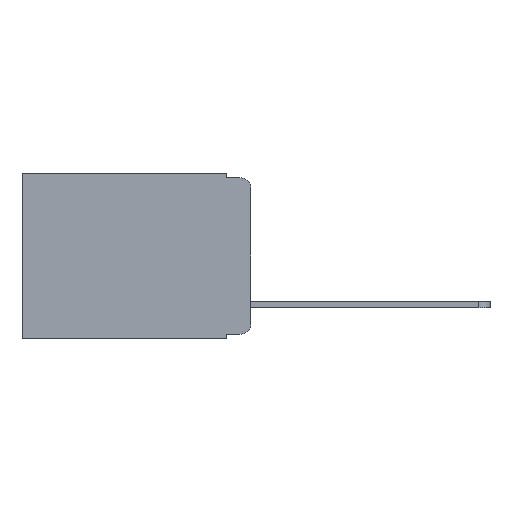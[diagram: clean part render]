
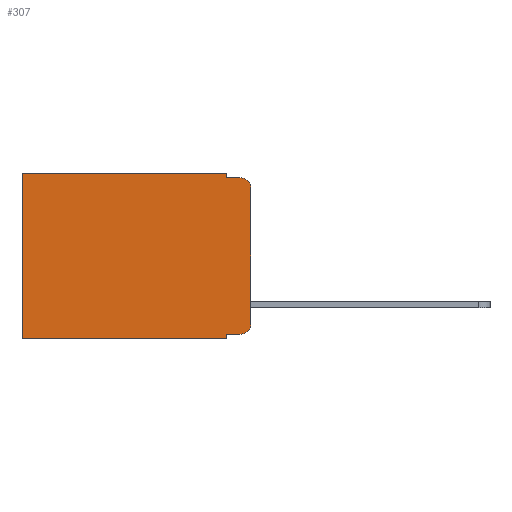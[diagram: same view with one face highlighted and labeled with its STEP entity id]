
A CAD part, left-side view. The second image highlights one B-rep face of the part: STEP entity #307.
In plain terms, the highlighted planar face has unit normal (-1, 0, 0).
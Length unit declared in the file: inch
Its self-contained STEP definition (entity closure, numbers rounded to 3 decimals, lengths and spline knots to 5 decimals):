
#84 = VERTEX_POINT ( 'NONE', #14097 ) ;
#109 = CARTESIAN_POINT ( 'NONE',  ( 0.298, 0.051, -0.01 ) ) ;
#186 = DIRECTION ( 'NONE',  ( 0., 0., -1. ) ) ;
#307 = ADVANCED_FACE ( 'NONE', ( #3112 ), #5571, .F. ) ;
#440 = VERTEX_POINT ( 'NONE', #2678 ) ;
#687 = CARTESIAN_POINT ( 'NONE',  ( 0.298, 0.051, -0.333 ) ) ;
#953 = AXIS2_PLACEMENT_3D ( 'NONE', #9244, #13733, #14903 ) ;
#974 = CARTESIAN_POINT ( 'NONE',  ( 0.298, 0., 0. ) ) ;
#1212 = DIRECTION ( 'NONE',  ( -1., 0., 0. ) ) ;
#1308 = EDGE_CURVE ( 'NONE', #11328, #84, #1599, .T. ) ;
#1599 = LINE ( 'NONE', #687, #10587 ) ;
#1631 = EDGE_CURVE ( 'NONE', #14155, #2158, #12744, .T. ) ;
#1841 = CARTESIAN_POINT ( 'NONE',  ( 0.298, 0.051, 0. ) ) ;
#2158 = VERTEX_POINT ( 'NONE', #7112 ) ;
#2267 = DIRECTION ( 'NONE',  ( 0., 1., 0. ) ) ;
#2623 = EDGE_LOOP ( 'NONE', ( #8849, #6569, #5108, #6076, #7747, #9225, #6138, #6035, #11601, #13265 ) ) ;
#2652 = CARTESIAN_POINT ( 'NONE',  ( 0.298, 0., -0.03 ) ) ;
#2678 = CARTESIAN_POINT ( 'NONE',  ( 0.298, 0.051, -0.01 ) ) ;
#2865 = VECTOR ( 'NONE', #2267, 39.37008 ) ;
#3112 = FACE_OUTER_BOUND ( 'NONE', #2623, .T. ) ;
#3610 = LINE ( 'NONE', #4688, #4541 ) ;
#3996 = EDGE_CURVE ( 'NONE', #10673, #12956, #5296, .T. ) ;
#4031 = VECTOR ( 'NONE', #14235, 39.37008 ) ;
#4123 = CARTESIAN_POINT ( 'NONE',  ( 0.298, 0., -0.313 ) ) ;
#4240 = VERTEX_POINT ( 'NONE', #4123 ) ;
#4541 = VECTOR ( 'NONE', #186, 39.37008 ) ;
#4688 = CARTESIAN_POINT ( 'NONE',  ( 0.298, 0.051, 0. ) ) ;
#4751 = EDGE_CURVE ( 'NONE', #11328, #10673, #3610, .T. ) ;
#4958 = EDGE_CURVE ( 'NONE', #12602, #440, #14024, .T. ) ;
#5108 = ORIENTED_EDGE ( 'NONE', *, *, #14728, .F. ) ;
#5249 = LINE ( 'NONE', #109, #7482 ) ;
#5296 = LINE ( 'NONE', #10644, #13701 ) ;
#5571 = PLANE ( 'NONE',  #953 ) ;
#5647 = CARTESIAN_POINT ( 'NONE',  ( 0.298, 0.051, 0. ) ) ;
#5767 = VECTOR ( 'NONE', #6922, 39.37008 ) ;
#5869 = CARTESIAN_POINT ( 'NONE',  ( 0.298, 0.02, -0.03 ) ) ;
#5973 = EDGE_CURVE ( 'NONE', #5981, #12956, #7658, .T. ) ;
#5981 = VERTEX_POINT ( 'NONE', #11500 ) ;
#6035 = ORIENTED_EDGE ( 'NONE', *, *, #4751, .F. ) ;
#6076 = ORIENTED_EDGE ( 'NONE', *, *, #4958, .F. ) ;
#6138 = ORIENTED_EDGE ( 'NONE', *, *, #3996, .F. ) ;
#6381 = EDGE_CURVE ( 'NONE', #12602, #5981, #12183, .T. ) ;
#6569 = ORIENTED_EDGE ( 'NONE', *, *, #1631, .T. ) ;
#6681 = AXIS2_PLACEMENT_3D ( 'NONE', #5869, #1212, #10533 ) ;
#6922 = DIRECTION ( 'NONE',  ( 0., 0., -1. ) ) ;
#6939 = CARTESIAN_POINT ( 'NONE',  ( 0.298, 0.473, -0.343 ) ) ;
#6941 = DIRECTION ( 'NONE',  ( 0., 0., -1. ) ) ;
#7038 = DIRECTION ( 'NONE',  ( 0., 1., 0. ) ) ;
#7112 = CARTESIAN_POINT ( 'NONE',  ( 0.298, 0.02, -0.01 ) ) ;
#7201 = DIRECTION ( 'NONE',  ( 0., -1., 0. ) ) ;
#7482 = VECTOR ( 'NONE', #7201, 39.37008 ) ;
#7658 = LINE ( 'NONE', #10441, #5767 ) ;
#7747 = ORIENTED_EDGE ( 'NONE', *, *, #6381, .T. ) ;
#8849 = ORIENTED_EDGE ( 'NONE', *, *, #11906, .F. ) ;
#9035 = DIRECTION ( 'NONE',  ( 0., 0., -1. ) ) ;
#9225 = ORIENTED_EDGE ( 'NONE', *, *, #5973, .T. ) ;
#9244 = CARTESIAN_POINT ( 'NONE',  ( 0.298, 0., 0. ) ) ;
#9601 = CARTESIAN_POINT ( 'NONE',  ( 0.298, 0.051, -0.343 ) ) ;
#10441 = CARTESIAN_POINT ( 'NONE',  ( 0.298, 0.473, 0. ) ) ;
#10533 = DIRECTION ( 'NONE',  ( 0., 0., -1. ) ) ;
#10587 = VECTOR ( 'NONE', #14777, 39.37008 ) ;
#10644 = CARTESIAN_POINT ( 'NONE',  ( 0.298, 0., -0.343 ) ) ;
#10673 = VERTEX_POINT ( 'NONE', #9601 ) ;
#11093 = AXIS2_PLACEMENT_3D ( 'NONE', #14982, #13907, #6941 ) ;
#11328 = VERTEX_POINT ( 'NONE', #13264 ) ;
#11500 = CARTESIAN_POINT ( 'NONE',  ( 0.298, 0.473, 0. ) ) ;
#11601 = ORIENTED_EDGE ( 'NONE', *, *, #1308, .T. ) ;
#11906 = EDGE_CURVE ( 'NONE', #14155, #4240, #12083, .T. ) ;
#12083 = LINE ( 'NONE', #14289, #4031 ) ;
#12183 = LINE ( 'NONE', #974, #2865 ) ;
#12602 = VERTEX_POINT ( 'NONE', #1841 ) ;
#12744 = CIRCLE ( 'NONE', #6681, 0.02 ) ;
#12956 = VERTEX_POINT ( 'NONE', #6939 ) ;
#13264 = CARTESIAN_POINT ( 'NONE',  ( 0.298, 0.051, -0.333 ) ) ;
#13265 = ORIENTED_EDGE ( 'NONE', *, *, #14576, .T. ) ;
#13701 = VECTOR ( 'NONE', #7038, 39.37008 ) ;
#13733 = DIRECTION ( 'NONE',  ( 1., 0., 0. ) ) ;
#13824 = CIRCLE ( 'NONE', #11093, 0.02 ) ;
#13907 = DIRECTION ( 'NONE',  ( -1., 0., 0. ) ) ;
#14024 = LINE ( 'NONE', #5647, #14750 ) ;
#14097 = CARTESIAN_POINT ( 'NONE',  ( 0.298, 0.02, -0.333 ) ) ;
#14155 = VERTEX_POINT ( 'NONE', #2652 ) ;
#14235 = DIRECTION ( 'NONE',  ( 0., 0., -1. ) ) ;
#14289 = CARTESIAN_POINT ( 'NONE',  ( 0.298, 0., 0. ) ) ;
#14576 = EDGE_CURVE ( 'NONE', #84, #4240, #13824, .T. ) ;
#14728 = EDGE_CURVE ( 'NONE', #440, #2158, #5249, .T. ) ;
#14750 = VECTOR ( 'NONE', #9035, 39.37008 ) ;
#14777 = DIRECTION ( 'NONE',  ( 0., -1., 0. ) ) ;
#14903 = DIRECTION ( 'NONE',  ( 0., 0., -1. ) ) ;
#14982 = CARTESIAN_POINT ( 'NONE',  ( 0.298, 0.02, -0.313 ) ) ;
